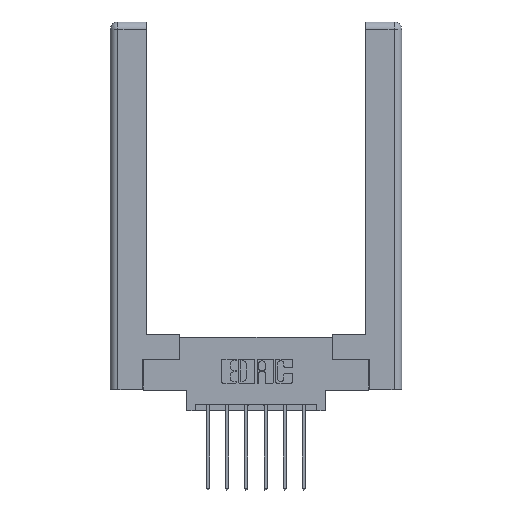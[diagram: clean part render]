
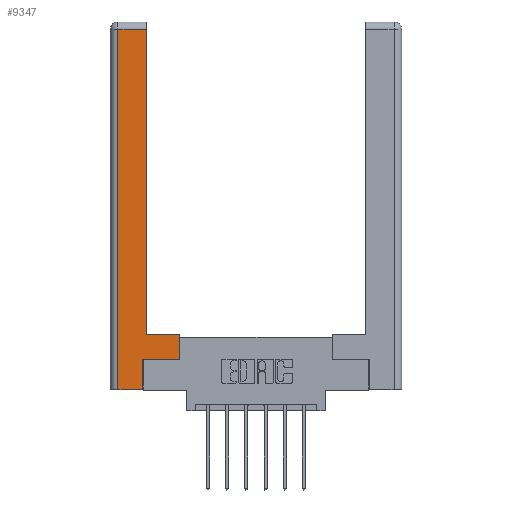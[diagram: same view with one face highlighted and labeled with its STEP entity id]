
A CAD part, top view. The second image highlights one B-rep face of the part: STEP entity #9347.
In plain terms, the highlighted planar face has unit normal (0, 0, 1).
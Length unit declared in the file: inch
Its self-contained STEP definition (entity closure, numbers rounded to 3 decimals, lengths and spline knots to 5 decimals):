
#11 = CARTESIAN_POINT ( 'NONE',  ( 0.265, 0.245, 0. ) ) ;
#184 = DIRECTION ( 'NONE',  ( -1., 0., 0. ) ) ;
#238 = ORIENTED_EDGE ( 'NONE', *, *, #9935, .T. ) ;
#419 = AXIS2_PLACEMENT_3D ( 'NONE', #6425, #10251, #8306 ) ;
#473 = ORIENTED_EDGE ( 'NONE', *, *, #3025, .T. ) ;
#742 = VECTOR ( 'NONE', #3442, 39.37008 ) ;
#791 = VERTEX_POINT ( 'NONE', #5975 ) ;
#864 = DIRECTION ( 'NONE',  ( 1., 0., 0. ) ) ;
#955 = CARTESIAN_POINT ( 'NONE',  ( 0.295, 2.94, 0. ) ) ;
#1560 = EDGE_CURVE ( 'NONE', #9017, #9334, #1907, .T. ) ;
#1907 = LINE ( 'NONE', #9906, #742 ) ;
#2106 = CARTESIAN_POINT ( 'NONE',  ( 0.295, 0.45, 0. ) ) ;
#2175 = DIRECTION ( 'NONE',  ( 0., -1., 0. ) ) ;
#2618 = ORIENTED_EDGE ( 'NONE', *, *, #2776, .T. ) ;
#2677 = CARTESIAN_POINT ( 'NONE',  ( 0.295, 3., 0. ) ) ;
#2684 = LINE ( 'NONE', #2106, #9723 ) ;
#2753 = CARTESIAN_POINT ( 'NONE',  ( 0.565, 0.45, 0. ) ) ;
#2776 = EDGE_CURVE ( 'NONE', #6275, #8892, #11687, .T. ) ;
#3025 = EDGE_CURVE ( 'NONE', #7640, #6275, #7270, .T. ) ;
#3165 = ORIENTED_EDGE ( 'NONE', *, *, #9344, .T. ) ;
#3198 = ORIENTED_EDGE ( 'NONE', *, *, #11268, .T. ) ;
#3202 = CARTESIAN_POINT ( 'NONE',  ( 0.565, 0.245, 0. ) ) ;
#3442 = DIRECTION ( 'NONE',  ( 0., 1., 0. ) ) ;
#3496 = VECTOR ( 'NONE', #2175, 39.37008 ) ;
#3567 = CARTESIAN_POINT ( 'NONE',  ( 0.565, 0.245, 0. ) ) ;
#3705 = PLANE ( 'NONE',  #419 ) ;
#3890 = VECTOR ( 'NONE', #9168, 39.37008 ) ;
#4424 = ORIENTED_EDGE ( 'NONE', *, *, #1560, .T. ) ;
#4548 = VERTEX_POINT ( 'NONE', #5382 ) ;
#4750 = LINE ( 'NONE', #2677, #3890 ) ;
#5382 = CARTESIAN_POINT ( 'NONE',  ( 0.265, 0., 0. ) ) ;
#5817 = CARTESIAN_POINT ( 'NONE',  ( 0.265, 0.245, 0. ) ) ;
#5975 = CARTESIAN_POINT ( 'NONE',  ( 0.295, 0.45, 0. ) ) ;
#5978 = VECTOR ( 'NONE', #6743, 39.37008 ) ;
#6275 = VERTEX_POINT ( 'NONE', #6401 ) ;
#6364 = LINE ( 'NONE', #11, #8424 ) ;
#6401 = CARTESIAN_POINT ( 'NONE',  ( 0.0615, 2.94, 0. ) ) ;
#6425 = CARTESIAN_POINT ( 'NONE',  ( 0., 0., 0. ) ) ;
#6743 = DIRECTION ( 'NONE',  ( -1., 0., 0. ) ) ;
#7270 = LINE ( 'NONE', #9702, #5978 ) ;
#7286 = DIRECTION ( 'NONE',  ( 0., 1., 0. ) ) ;
#7640 = VERTEX_POINT ( 'NONE', #955 ) ;
#7726 = EDGE_LOOP ( 'NONE', ( #3165, #473, #2618, #3198, #12085, #238, #4424, #10895 ) ) ;
#7739 = CARTESIAN_POINT ( 'NONE',  ( 0.0615, 0., 0. ) ) ;
#7841 = CARTESIAN_POINT ( 'NONE',  ( 0.0615, 0., 0. ) ) ;
#8306 = DIRECTION ( 'NONE',  ( -1., 0., 0. ) ) ;
#8328 = CARTESIAN_POINT ( 'NONE',  ( 0.265, 0., 0. ) ) ;
#8424 = VECTOR ( 'NONE', #7286, 39.37008 ) ;
#8695 = LINE ( 'NONE', #8328, #10305 ) ;
#8892 = VERTEX_POINT ( 'NONE', #7841 ) ;
#9017 = VERTEX_POINT ( 'NONE', #3567 ) ;
#9168 = DIRECTION ( 'NONE',  ( 0., 1., 0. ) ) ;
#9334 = VERTEX_POINT ( 'NONE', #2753 ) ;
#9344 = EDGE_CURVE ( 'NONE', #791, #7640, #4750, .T. ) ;
#9347 = ADVANCED_FACE ( 'NONE', ( #10339 ), #3705, .F. ) ;
#9408 = EDGE_CURVE ( 'NONE', #4548, #10579, #6364, .T. ) ;
#9702 = CARTESIAN_POINT ( 'NONE',  ( 0.0615, 2.94, 0. ) ) ;
#9723 = VECTOR ( 'NONE', #184, 39.37008 ) ;
#9906 = CARTESIAN_POINT ( 'NONE',  ( 0.565, 0.45, 0. ) ) ;
#9935 = EDGE_CURVE ( 'NONE', #10579, #9017, #11638, .T. ) ;
#10191 = VECTOR ( 'NONE', #10554, 39.37008 ) ;
#10251 = DIRECTION ( 'NONE',  ( 0., 0., -1. ) ) ;
#10305 = VECTOR ( 'NONE', #864, 39.37008 ) ;
#10339 = FACE_OUTER_BOUND ( 'NONE', #7726, .T. ) ;
#10554 = DIRECTION ( 'NONE',  ( 1., 0., 0. ) ) ;
#10579 = VERTEX_POINT ( 'NONE', #5817 ) ;
#10895 = ORIENTED_EDGE ( 'NONE', *, *, #11332, .T. ) ;
#11268 = EDGE_CURVE ( 'NONE', #8892, #4548, #8695, .T. ) ;
#11332 = EDGE_CURVE ( 'NONE', #9334, #791, #2684, .T. ) ;
#11638 = LINE ( 'NONE', #3202, #10191 ) ;
#11687 = LINE ( 'NONE', #7739, #3496 ) ;
#12085 = ORIENTED_EDGE ( 'NONE', *, *, #9408, .T. ) ;
